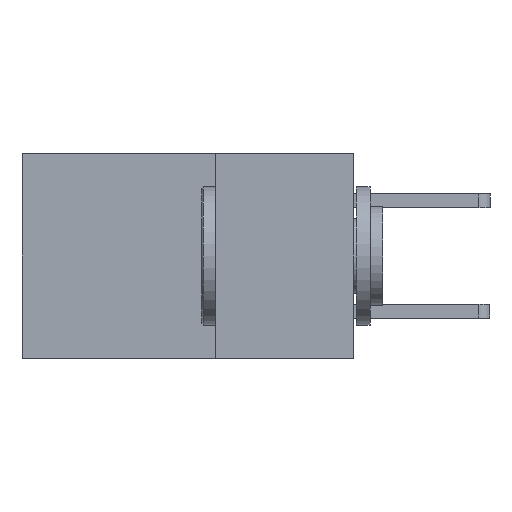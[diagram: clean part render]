
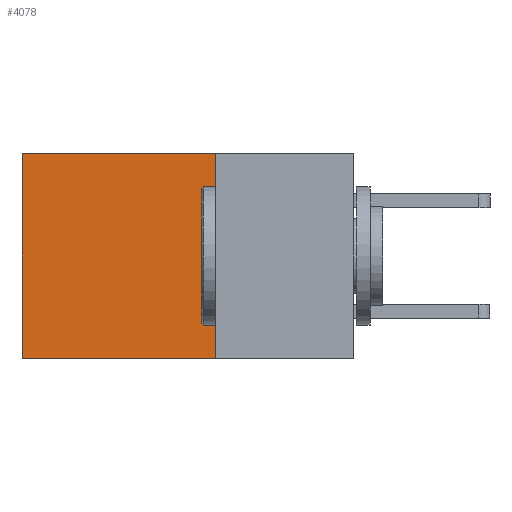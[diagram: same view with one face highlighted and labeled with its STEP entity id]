
A CAD part, left-side view. The second image highlights one B-rep face of the part: STEP entity #4078.
In plain terms, the highlighted planar face has unit normal (-1, 0, 0).
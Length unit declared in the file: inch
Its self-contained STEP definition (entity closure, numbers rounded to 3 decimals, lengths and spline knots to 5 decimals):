
#39 = CARTESIAN_POINT ( 'NONE',  ( 0.2875, 0.25, -0.37 ) ) ;
#361 = DIRECTION ( 'NONE',  ( 0., 1., 0. ) ) ;
#468 = ORIENTED_EDGE ( 'NONE', *, *, #6183, .T. ) ;
#1198 = CARTESIAN_POINT ( 'NONE',  ( 0.2875, 0.25, -0.37 ) ) ;
#1222 = CARTESIAN_POINT ( 'NONE',  ( 0.2875, 0.25, 0. ) ) ;
#1566 = VERTEX_POINT ( 'NONE', #5473 ) ;
#2390 = DIRECTION ( 'NONE',  ( 0., 0., -1. ) ) ;
#2781 = VECTOR ( 'NONE', #361, 39.37008 ) ;
#3308 = AXIS2_PLACEMENT_3D ( 'NONE', #1222, #11751, #9497 ) ;
#3830 = LINE ( 'NONE', #11222, #8832 ) ;
#4078 = ADVANCED_FACE ( 'NONE', ( #10826 ), #6771, .F. ) ;
#4366 = LINE ( 'NONE', #10774, #6067 ) ;
#4603 = VERTEX_POINT ( 'NONE', #1198 ) ;
#4836 = EDGE_CURVE ( 'NONE', #9504, #1566, #3830, .T. ) ;
#4948 = ORIENTED_EDGE ( 'NONE', *, *, #4836, .T. ) ;
#5473 = CARTESIAN_POINT ( 'NONE',  ( 0.2875, 0.6, -0.37 ) ) ;
#5997 = VERTEX_POINT ( 'NONE', #10282 ) ;
#6067 = VECTOR ( 'NONE', #2390, 39.37008 ) ;
#6183 = EDGE_CURVE ( 'NONE', #5997, #9504, #8831, .T. ) ;
#6771 = PLANE ( 'NONE',  #3308 ) ;
#8831 = LINE ( 'NONE', #10528, #2781 ) ;
#8832 = VECTOR ( 'NONE', #11344, 39.37008 ) ;
#9238 = DIRECTION ( 'NONE',  ( 0., 1., 0. ) ) ;
#9497 = DIRECTION ( 'NONE',  ( 0., 0., -1. ) ) ;
#9504 = VERTEX_POINT ( 'NONE', #11001 ) ;
#9565 = EDGE_LOOP ( 'NONE', ( #4948, #11411, #12022, #468 ) ) ;
#10282 = CARTESIAN_POINT ( 'NONE',  ( 0.2875, 0.25, 0. ) ) ;
#10297 = EDGE_CURVE ( 'NONE', #5997, #4603, #4366, .T. ) ;
#10502 = EDGE_CURVE ( 'NONE', #4603, #1566, #11077, .T. ) ;
#10528 = CARTESIAN_POINT ( 'NONE',  ( 0.2875, 0.25, 0. ) ) ;
#10735 = VECTOR ( 'NONE', #9238, 39.37008 ) ;
#10774 = CARTESIAN_POINT ( 'NONE',  ( 0.2875, 0.25, 0. ) ) ;
#10826 = FACE_OUTER_BOUND ( 'NONE', #9565, .T. ) ;
#11001 = CARTESIAN_POINT ( 'NONE',  ( 0.2875, 0.6, 0. ) ) ;
#11077 = LINE ( 'NONE', #39, #10735 ) ;
#11222 = CARTESIAN_POINT ( 'NONE',  ( 0.2875, 0.6, 0. ) ) ;
#11344 = DIRECTION ( 'NONE',  ( 0., 0., -1. ) ) ;
#11411 = ORIENTED_EDGE ( 'NONE', *, *, #10502, .F. ) ;
#11751 = DIRECTION ( 'NONE',  ( 1., 0., 0. ) ) ;
#12022 = ORIENTED_EDGE ( 'NONE', *, *, #10297, .F. ) ;
